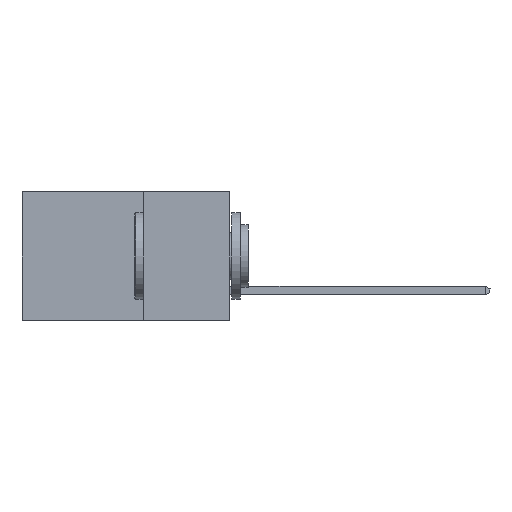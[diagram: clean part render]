
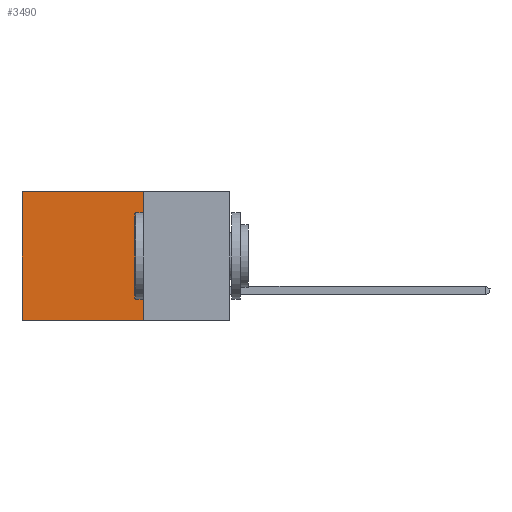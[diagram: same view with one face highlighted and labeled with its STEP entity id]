
A CAD part, left-side view. The second image highlights one B-rep face of the part: STEP entity #3490.
In plain terms, the highlighted planar face has unit normal (-1, 0, 0).
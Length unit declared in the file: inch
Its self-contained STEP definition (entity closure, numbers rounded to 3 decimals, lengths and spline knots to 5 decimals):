
#896 = DIRECTION ( 'NONE',  ( 0., 0., -1. ) ) ;
#1040 = ORIENTED_EDGE ( 'NONE', *, *, #7158, .T. ) ;
#1657 = DIRECTION ( 'NONE',  ( 0., 0., -1. ) ) ;
#1748 = DIRECTION ( 'NONE',  ( 0., 0., -1. ) ) ;
#2377 = LINE ( 'NONE', #6552, #5614 ) ;
#2489 = CARTESIAN_POINT ( 'NONE',  ( 0.2615, 0.6, -0.37 ) ) ;
#2510 = FACE_OUTER_BOUND ( 'NONE', #11407, .T. ) ;
#2897 = EDGE_CURVE ( 'NONE', #9514, #3194, #5757, .T. ) ;
#2933 = ORIENTED_EDGE ( 'NONE', *, *, #2897, .F. ) ;
#3194 = VERTEX_POINT ( 'NONE', #5815 ) ;
#3417 = LINE ( 'NONE', #10034, #8847 ) ;
#3436 = EDGE_CURVE ( 'NONE', #3194, #11431, #3417, .T. ) ;
#3490 = ADVANCED_FACE ( 'NONE', ( #2510 ), #7586, .F. ) ;
#4613 = DIRECTION ( 'NONE',  ( 0., 1., 0. ) ) ;
#4824 = ORIENTED_EDGE ( 'NONE', *, *, #8845, .T. ) ;
#5292 = VERTEX_POINT ( 'NONE', #11484 ) ;
#5602 = DIRECTION ( 'NONE',  ( 1., 0., 0. ) ) ;
#5614 = VECTOR ( 'NONE', #1657, 39.37008 ) ;
#5757 = LINE ( 'NONE', #9685, #7662 ) ;
#5815 = CARTESIAN_POINT ( 'NONE',  ( 0.2615, 0.25, -0.37 ) ) ;
#6552 = CARTESIAN_POINT ( 'NONE',  ( 0.2615, 0.6, -0.37 ) ) ;
#6801 = AXIS2_PLACEMENT_3D ( 'NONE', #8559, #5602, #1748 ) ;
#7158 = EDGE_CURVE ( 'NONE', #5292, #11431, #2377, .T. ) ;
#7396 = CARTESIAN_POINT ( 'NONE',  ( 0.2615, 0.25, 0. ) ) ;
#7586 = PLANE ( 'NONE',  #6801 ) ;
#7662 = VECTOR ( 'NONE', #896, 39.37008 ) ;
#7898 = VECTOR ( 'NONE', #4613, 39.37008 ) ;
#8559 = CARTESIAN_POINT ( 'NONE',  ( 0.2615, 0.25, -0.37 ) ) ;
#8845 = EDGE_CURVE ( 'NONE', #9514, #5292, #10393, .T. ) ;
#8847 = VECTOR ( 'NONE', #12015, 39.37008 ) ;
#9514 = VERTEX_POINT ( 'NONE', #7396 ) ;
#9685 = CARTESIAN_POINT ( 'NONE',  ( 0.2615, 0.25, -0.37 ) ) ;
#10034 = CARTESIAN_POINT ( 'NONE',  ( 0.2615, 0.25, -0.37 ) ) ;
#10393 = LINE ( 'NONE', #10449, #7898 ) ;
#10449 = CARTESIAN_POINT ( 'NONE',  ( 0.2615, 0.25, 0. ) ) ;
#11407 = EDGE_LOOP ( 'NONE', ( #1040, #12630, #2933, #4824 ) ) ;
#11431 = VERTEX_POINT ( 'NONE', #2489 ) ;
#11484 = CARTESIAN_POINT ( 'NONE',  ( 0.2615, 0.6, 0. ) ) ;
#12015 = DIRECTION ( 'NONE',  ( 0., 1., 0. ) ) ;
#12630 = ORIENTED_EDGE ( 'NONE', *, *, #3436, .F. ) ;
